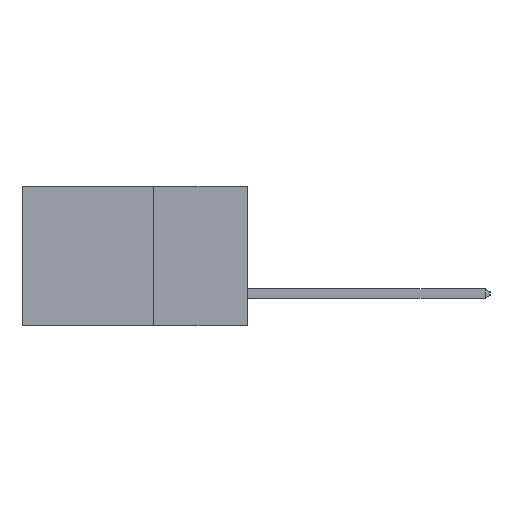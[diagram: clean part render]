
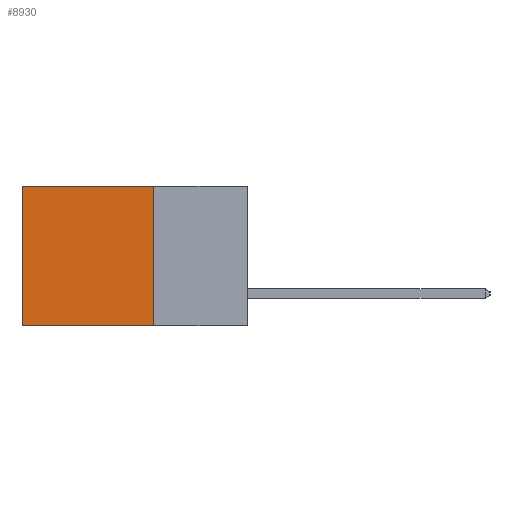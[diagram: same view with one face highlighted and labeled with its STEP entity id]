
A CAD part, left-side view. The second image highlights one B-rep face of the part: STEP entity #8930.
In plain terms, the highlighted planar face has unit normal (-1, 0, 0).
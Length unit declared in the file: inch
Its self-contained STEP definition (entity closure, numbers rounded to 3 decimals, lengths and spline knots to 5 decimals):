
#1024 = VERTEX_POINT ( 'NONE', #9020 ) ;
#1380 = ORIENTED_EDGE ( 'NONE', *, *, #4690, .T. ) ;
#1518 = VECTOR ( 'NONE', #13058, 39.37008 ) ;
#1615 = DIRECTION ( 'NONE',  ( 0., 1., 0. ) ) ;
#2209 = VECTOR ( 'NONE', #22919, 39.37008 ) ;
#2456 = VERTEX_POINT ( 'NONE', #9251 ) ;
#2810 = LINE ( 'NONE', #3253, #2209 ) ;
#3253 = CARTESIAN_POINT ( 'NONE',  ( 0.2615, 0.6, -0.37 ) ) ;
#3849 = LINE ( 'NONE', #15855, #9135 ) ;
#4690 = EDGE_CURVE ( 'NONE', #10412, #2456, #3849, .T. ) ;
#6123 = FACE_OUTER_BOUND ( 'NONE', #7558, .T. ) ;
#6790 = VERTEX_POINT ( 'NONE', #13672 ) ;
#6798 = LINE ( 'NONE', #13031, #1518 ) ;
#6932 = EDGE_CURVE ( 'NONE', #10412, #1024, #6798, .T. ) ;
#7548 = ORIENTED_EDGE ( 'NONE', *, *, #6932, .F. ) ;
#7558 = EDGE_LOOP ( 'NONE', ( #21320, #9806, #7548, #1380 ) ) ;
#8930 = ADVANCED_FACE ( 'NONE', ( #6123 ), #11256, .F. ) ;
#9020 = CARTESIAN_POINT ( 'NONE',  ( 0.2615, 0.25, -0.37 ) ) ;
#9135 = VECTOR ( 'NONE', #16121, 39.37008 ) ;
#9251 = CARTESIAN_POINT ( 'NONE',  ( 0.2615, 0.6, 0. ) ) ;
#9806 = ORIENTED_EDGE ( 'NONE', *, *, #16597, .F. ) ;
#10412 = VERTEX_POINT ( 'NONE', #11978 ) ;
#10635 = DIRECTION ( 'NONE',  ( 0., 0., -1. ) ) ;
#10849 = VECTOR ( 'NONE', #1615, 39.37008 ) ;
#10851 = DIRECTION ( 'NONE',  ( 1., 0., 0. ) ) ;
#10939 = CARTESIAN_POINT ( 'NONE',  ( 0.2615, 0.25, -0.37 ) ) ;
#11256 = PLANE ( 'NONE',  #21233 ) ;
#11978 = CARTESIAN_POINT ( 'NONE',  ( 0.2615, 0.25, 0. ) ) ;
#13031 = CARTESIAN_POINT ( 'NONE',  ( 0.2615, 0.25, -0.37 ) ) ;
#13058 = DIRECTION ( 'NONE',  ( 0., 0., -1. ) ) ;
#13672 = CARTESIAN_POINT ( 'NONE',  ( 0.2615, 0.6, -0.37 ) ) ;
#15855 = CARTESIAN_POINT ( 'NONE',  ( 0.2615, 0.25, 0. ) ) ;
#16121 = DIRECTION ( 'NONE',  ( 0., 1., 0. ) ) ;
#16505 = EDGE_CURVE ( 'NONE', #2456, #6790, #2810, .T. ) ;
#16597 = EDGE_CURVE ( 'NONE', #1024, #6790, #20708, .T. ) ;
#20708 = LINE ( 'NONE', #23251, #10849 ) ;
#21233 = AXIS2_PLACEMENT_3D ( 'NONE', #10939, #10851, #10635 ) ;
#21320 = ORIENTED_EDGE ( 'NONE', *, *, #16505, .T. ) ;
#22919 = DIRECTION ( 'NONE',  ( 0., 0., -1. ) ) ;
#23251 = CARTESIAN_POINT ( 'NONE',  ( 0.2615, 0.25, -0.37 ) ) ;
